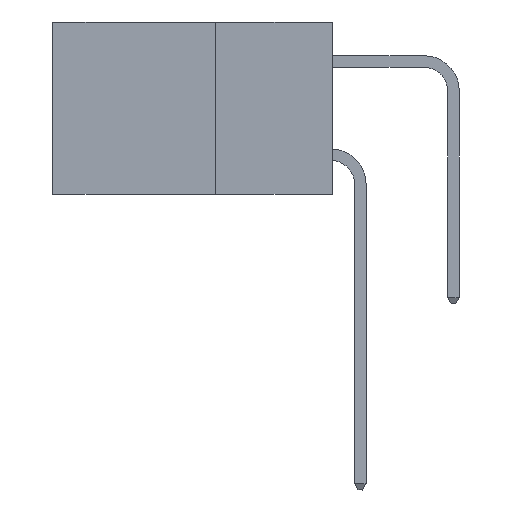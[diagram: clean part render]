
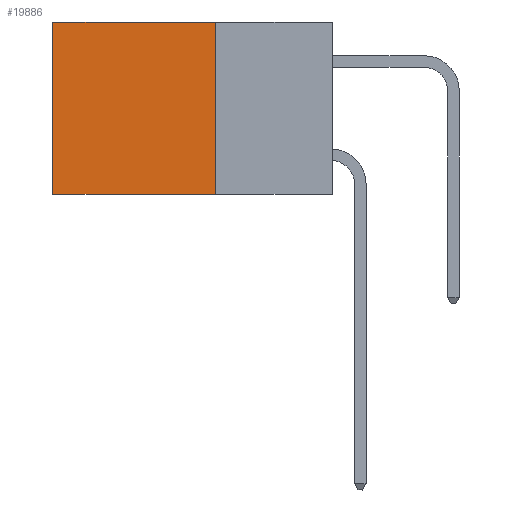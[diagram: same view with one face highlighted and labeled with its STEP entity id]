
A CAD part, left-side view. The second image highlights one B-rep face of the part: STEP entity #19886.
In plain terms, the highlighted planar face has unit normal (-1, 0, 0).
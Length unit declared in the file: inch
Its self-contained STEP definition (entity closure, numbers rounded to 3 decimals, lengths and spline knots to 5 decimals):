
#1063 = FACE_OUTER_BOUND ( 'NONE', #7214, .T. ) ;
#1530 = VECTOR ( 'NONE', #14702, 39.37008 ) ;
#1696 = CARTESIAN_POINT ( 'NONE',  ( 0.298, 0.25, -0.37 ) ) ;
#2097 = EDGE_CURVE ( 'NONE', #19570, #19344, #4830, .T. ) ;
#2102 = DIRECTION ( 'NONE',  ( 0., 0., -1. ) ) ;
#2718 = LINE ( 'NONE', #21008, #17195 ) ;
#3340 = AXIS2_PLACEMENT_3D ( 'NONE', #19607, #17690, #2102 ) ;
#3610 = CARTESIAN_POINT ( 'NONE',  ( 0.298, 0.25, -0.37 ) ) ;
#4830 = LINE ( 'NONE', #13191, #1530 ) ;
#4916 = LINE ( 'NONE', #1696, #12544 ) ;
#4999 = VERTEX_POINT ( 'NONE', #12476 ) ;
#7040 = DIRECTION ( 'NONE',  ( 0., 1., 0. ) ) ;
#7181 = ORIENTED_EDGE ( 'NONE', *, *, #22314, .F. ) ;
#7214 = EDGE_LOOP ( 'NONE', ( #17456, #7181, #7316, #16833 ) ) ;
#7316 = ORIENTED_EDGE ( 'NONE', *, *, #7905, .F. ) ;
#7905 = EDGE_CURVE ( 'NONE', #4999, #19467, #2718, .T. ) ;
#10300 = CARTESIAN_POINT ( 'NONE',  ( 0.298, 0.6, -0.37 ) ) ;
#10517 = DIRECTION ( 'NONE',  ( 0., 0., -1. ) ) ;
#10537 = DIRECTION ( 'NONE',  ( 0., 1., 0. ) ) ;
#11247 = CARTESIAN_POINT ( 'NONE',  ( 0.298, 0.6, 0. ) ) ;
#12476 = CARTESIAN_POINT ( 'NONE',  ( 0.298, 0.25, 0. ) ) ;
#12544 = VECTOR ( 'NONE', #7040, 39.37008 ) ;
#12571 = LINE ( 'NONE', #17653, #19104 ) ;
#13191 = CARTESIAN_POINT ( 'NONE',  ( 0.298, 0.6, 0. ) ) ;
#14702 = DIRECTION ( 'NONE',  ( 0., 0., -1. ) ) ;
#16833 = ORIENTED_EDGE ( 'NONE', *, *, #21990, .T. ) ;
#17195 = VECTOR ( 'NONE', #10517, 39.37008 ) ;
#17456 = ORIENTED_EDGE ( 'NONE', *, *, #2097, .T. ) ;
#17554 = PLANE ( 'NONE',  #3340 ) ;
#17653 = CARTESIAN_POINT ( 'NONE',  ( 0.298, 0.25, 0. ) ) ;
#17690 = DIRECTION ( 'NONE',  ( 1., 0., 0. ) ) ;
#19104 = VECTOR ( 'NONE', #10537, 39.37008 ) ;
#19344 = VERTEX_POINT ( 'NONE', #10300 ) ;
#19467 = VERTEX_POINT ( 'NONE', #3610 ) ;
#19570 = VERTEX_POINT ( 'NONE', #11247 ) ;
#19607 = CARTESIAN_POINT ( 'NONE',  ( 0.298, 0.25, 0. ) ) ;
#19886 = ADVANCED_FACE ( 'NONE', ( #1063 ), #17554, .F. ) ;
#21008 = CARTESIAN_POINT ( 'NONE',  ( 0.298, 0.25, 0. ) ) ;
#21990 = EDGE_CURVE ( 'NONE', #4999, #19570, #12571, .T. ) ;
#22314 = EDGE_CURVE ( 'NONE', #19467, #19344, #4916, .T. ) ;
